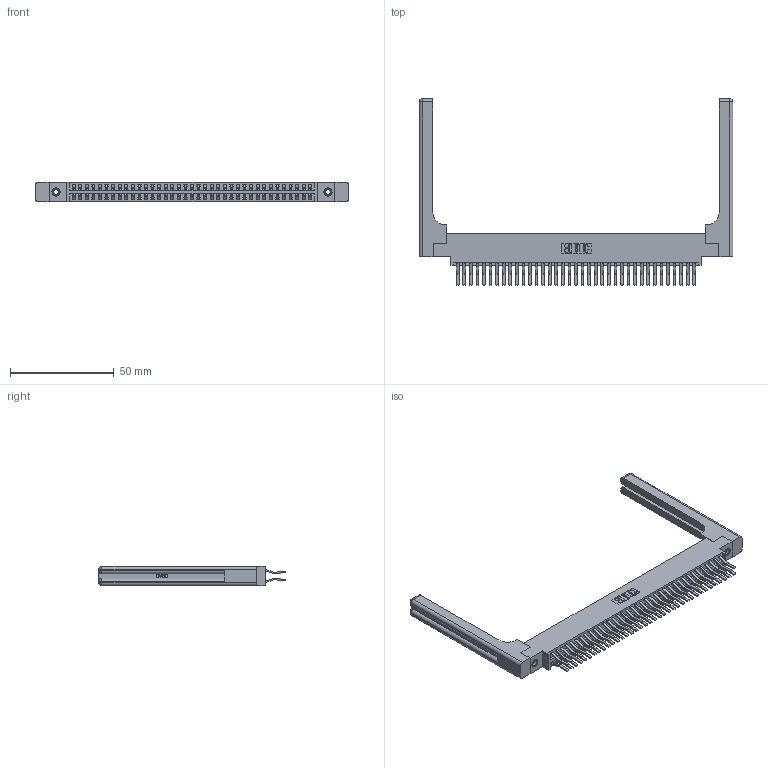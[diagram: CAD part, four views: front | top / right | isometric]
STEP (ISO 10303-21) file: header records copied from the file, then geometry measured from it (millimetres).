
FILE_DESCRIPTION (( 'STEP AP203' ), '1' );
FILE_NAME ('396-074-560-858.STEP', '2019-11-02T12:49:01', ( '' ), ( '' ), 'SwSTEP 2.0', 'SolidWorks 2016', '' );
FILE_SCHEMA (( 'CONFIG_CONTROL_DESIGN' ));
Length unit declared in the file: inch
Products named in the file (5): 345-250-001_345-250-001-102; 346-220-058_345-220-058; 396-074-560-858; 346 Part_0.170 Offset - 0.156 Dia-TH; 345-292-001_560 Tail
Assembly tree (79 placements, depth 2):
  396-074-560-858
    346 Part_0.170 Offset - 0.156 Dia-TH
    345-292-001_560 Tail  x74
    345-250-001_345-250-001-102  x2
    346-220-058_345-220-058  x2
Bounding box: 151.54 x 90.05 x 9.4 mm (x, y, z)
Volume: 22562.5 mm3; surface area: 27080.2 mm2
Topology: 79 solids, 79 shells, 4378 faces, 12921 edges, 8494 vertices
Faces by surface type: plane 2818, cylinder 1500, bspline 36, cone 12, sphere 8, torus 4
Entity records: 30222 total; most frequent: CARTESIAN_POINT 5997, ORIENTED_EDGE 4728, DIRECTION 4272, EDGE_CURVE 2364, VECTOR 1988, LINE 1988, VERTEX_POINT 1566, AXIS2_PLACEMENT_3D 1142
